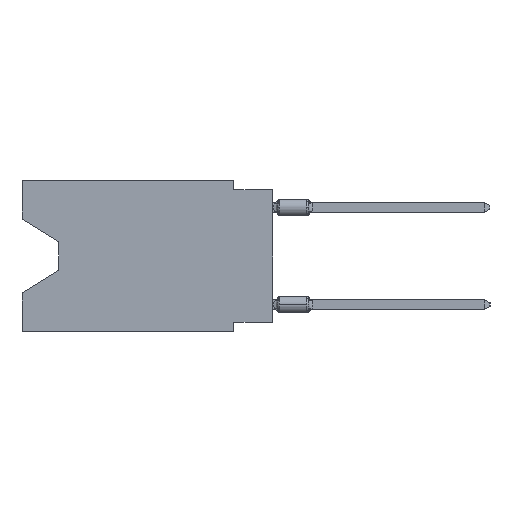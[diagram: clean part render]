
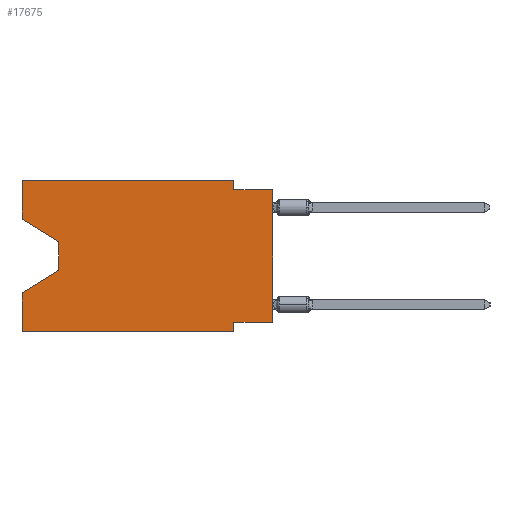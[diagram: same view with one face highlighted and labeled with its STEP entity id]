
A CAD part, left-side view. The second image highlights one B-rep face of the part: STEP entity #17675.
In plain terms, the highlighted planar face has unit normal (-1, 0, 0).
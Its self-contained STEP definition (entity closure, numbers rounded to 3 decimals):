
#400 = CARTESIAN_POINT ( 'NONE',  ( 0., 16.383, -7.36 ) ) ;
#507 = CARTESIAN_POINT ( 'NONE',  ( 0., 16.383, -2.546 ) ) ;
#830 = CARTESIAN_POINT ( 'NONE',  ( 0., 16.383, 0. ) ) ;
#953 = CARTESIAN_POINT ( 'NONE',  ( 0., 0., -0.635 ) ) ;
#1792 = VERTEX_POINT ( 'NONE', #2615 ) ;
#1834 = LINE ( 'NONE', #24312, #50578 ) ;
#1923 = ORIENTED_EDGE ( 'NONE', *, *, #20332, .F. ) ;
#2048 = LINE ( 'NONE', #46701, #47165 ) ;
#2173 = CARTESIAN_POINT ( 'NONE',  ( 0., 13.97, -5.893 ) ) ;
#2421 = VERTEX_POINT ( 'NONE', #4328 ) ;
#2615 = CARTESIAN_POINT ( 'NONE',  ( 0., 16.383, 0. ) ) ;
#3046 = LINE ( 'NONE', #54274, #6098 ) ;
#3304 = VERTEX_POINT ( 'NONE', #55934 ) ;
#4238 = DIRECTION ( 'NONE',  ( 0., 0., -1. ) ) ;
#4328 = CARTESIAN_POINT ( 'NONE',  ( 0., 2.54, -9.271 ) ) ;
#4760 = DIRECTION ( 'NONE',  ( 0., 0., 1. ) ) ;
#5270 = EDGE_CURVE ( 'NONE', #3304, #9733, #3046, .T. ) ;
#6098 = VECTOR ( 'NONE', #26111, 1000. ) ;
#6349 = EDGE_CURVE ( 'NONE', #2421, #26144, #16828, .T. ) ;
#6357 = CARTESIAN_POINT ( 'NONE',  ( 0., 2.54, -9.906 ) ) ;
#8248 = CARTESIAN_POINT ( 'NONE',  ( 0., 16.383, -9.906 ) ) ;
#8907 = EDGE_CURVE ( 'NONE', #13783, #26144, #40299, .T. ) ;
#9733 = VERTEX_POINT ( 'NONE', #2173 ) ;
#11800 = EDGE_CURVE ( 'NONE', #40457, #2421, #2048, .T. ) ;
#12446 = DIRECTION ( 'NONE',  ( 0., -1., 0. ) ) ;
#13056 = CARTESIAN_POINT ( 'NONE',  ( 0., 0., -9.271 ) ) ;
#13783 = VERTEX_POINT ( 'NONE', #56507 ) ;
#14037 = CARTESIAN_POINT ( 'NONE',  ( 0., 16.383, 0. ) ) ;
#14613 = PLANE ( 'NONE',  #41885 ) ;
#14623 = LINE ( 'NONE', #14037, #58030 ) ;
#14653 = DIRECTION ( 'NONE',  ( 0., 1., 0. ) ) ;
#14740 = VERTEX_POINT ( 'NONE', #26604 ) ;
#14767 = VECTOR ( 'NONE', #42408, 1000. ) ;
#15304 = DIRECTION ( 'NONE',  ( 0., 0., 1. ) ) ;
#15509 = EDGE_CURVE ( 'NONE', #1792, #32049, #58820, .T. ) ;
#15875 = CARTESIAN_POINT ( 'NONE',  ( 0., 16.383, 0. ) ) ;
#16316 = VERTEX_POINT ( 'NONE', #26539 ) ;
#16598 = LINE ( 'NONE', #26487, #50656 ) ;
#16828 = LINE ( 'NONE', #25527, #14767 ) ;
#17108 = CARTESIAN_POINT ( 'NONE',  ( 0., 2.54, 0. ) ) ;
#17675 = ADVANCED_FACE ( 'NONE', ( #46363 ), #14613, .F. ) ;
#18218 = DIRECTION ( 'NONE',  ( 0., 0., -1. ) ) ;
#19135 = VECTOR ( 'NONE', #34436, 1000. ) ;
#19222 = DIRECTION ( 'NONE',  ( 0., -1., 0. ) ) ;
#19463 = EDGE_CURVE ( 'NONE', #9733, #44950, #16598, .T. ) ;
#20332 = EDGE_CURVE ( 'NONE', #26983, #1792, #43433, .T. ) ;
#21745 = ORIENTED_EDGE ( 'NONE', *, *, #48545, .F. ) ;
#23669 = EDGE_CURVE ( 'NONE', #40457, #14740, #1834, .T. ) ;
#24005 = EDGE_LOOP ( 'NONE', ( #36872, #46896, #35415, #21745, #49447, #27276, #43816, #47415, #53205, #27104, #34881, #1923 ) ) ;
#24312 = CARTESIAN_POINT ( 'NONE',  ( 0., 0., 0. ) ) ;
#25527 = CARTESIAN_POINT ( 'NONE',  ( 0., 2.54, -9.906 ) ) ;
#25591 = DIRECTION ( 'NONE',  ( 0., 0.855, -0.519 ) ) ;
#26111 = DIRECTION ( 'NONE',  ( 0., 0., -1. ) ) ;
#26144 = VERTEX_POINT ( 'NONE', #6357 ) ;
#26487 = CARTESIAN_POINT ( 'NONE',  ( 0., 13.97, -5.893 ) ) ;
#26539 = CARTESIAN_POINT ( 'NONE',  ( 0., 2.54, -0.635 ) ) ;
#26604 = CARTESIAN_POINT ( 'NONE',  ( 0., 0., -0.635 ) ) ;
#26983 = VERTEX_POINT ( 'NONE', #42974 ) ;
#27002 = LINE ( 'NONE', #17108, #46323 ) ;
#27104 = ORIENTED_EDGE ( 'NONE', *, *, #31969, .F. ) ;
#27276 = ORIENTED_EDGE ( 'NONE', *, *, #6349, .F. ) ;
#27596 = CARTESIAN_POINT ( 'NONE',  ( 0., 2.54, 0. ) ) ;
#31969 = EDGE_CURVE ( 'NONE', #32049, #16316, #27002, .T. ) ;
#32049 = VERTEX_POINT ( 'NONE', #27596 ) ;
#32718 = VECTOR ( 'NONE', #12446, 1000. ) ;
#34436 = DIRECTION ( 'NONE',  ( 0., 0., 1. ) ) ;
#34837 = CARTESIAN_POINT ( 'NONE',  ( 0., 16.383, 0. ) ) ;
#34881 = ORIENTED_EDGE ( 'NONE', *, *, #15509, .F. ) ;
#35113 = VECTOR ( 'NONE', #58217, 1000. ) ;
#35415 = ORIENTED_EDGE ( 'NONE', *, *, #19463, .T. ) ;
#36872 = ORIENTED_EDGE ( 'NONE', *, *, #42463, .T. ) ;
#40299 = LINE ( 'NONE', #8248, #32718 ) ;
#40457 = VERTEX_POINT ( 'NONE', #13056 ) ;
#41560 = LINE ( 'NONE', #507, #48141 ) ;
#41885 = AXIS2_PLACEMENT_3D ( 'NONE', #830, #54481, #18218 ) ;
#42408 = DIRECTION ( 'NONE',  ( 0., 0., -1. ) ) ;
#42463 = EDGE_CURVE ( 'NONE', #26983, #3304, #41560, .T. ) ;
#42974 = CARTESIAN_POINT ( 'NONE',  ( 0., 16.383, -2.546 ) ) ;
#43433 = LINE ( 'NONE', #15875, #19135 ) ;
#43816 = ORIENTED_EDGE ( 'NONE', *, *, #11800, .F. ) ;
#44950 = VERTEX_POINT ( 'NONE', #400 ) ;
#46323 = VECTOR ( 'NONE', #4238, 1000. ) ;
#46363 = FACE_OUTER_BOUND ( 'NONE', #24005, .T. ) ;
#46701 = CARTESIAN_POINT ( 'NONE',  ( 0., 0., -9.271 ) ) ;
#46770 = LINE ( 'NONE', #953, #49103 ) ;
#46896 = ORIENTED_EDGE ( 'NONE', *, *, #5270, .T. ) ;
#47165 = VECTOR ( 'NONE', #14653, 1000. ) ;
#47415 = ORIENTED_EDGE ( 'NONE', *, *, #23669, .T. ) ;
#48141 = VECTOR ( 'NONE', #51423, 1000. ) ;
#48545 = EDGE_CURVE ( 'NONE', #13783, #44950, #14623, .T. ) ;
#49103 = VECTOR ( 'NONE', #19222, 1000. ) ;
#49447 = ORIENTED_EDGE ( 'NONE', *, *, #8907, .T. ) ;
#50578 = VECTOR ( 'NONE', #15304, 1000. ) ;
#50656 = VECTOR ( 'NONE', #25591, 1000. ) ;
#51423 = DIRECTION ( 'NONE',  ( 0., -0.855, -0.519 ) ) ;
#52848 = EDGE_CURVE ( 'NONE', #16316, #14740, #46770, .T. ) ;
#53205 = ORIENTED_EDGE ( 'NONE', *, *, #52848, .F. ) ;
#54274 = CARTESIAN_POINT ( 'NONE',  ( 0., 13.97, -4.013 ) ) ;
#54481 = DIRECTION ( 'NONE',  ( 1., 0., 0. ) ) ;
#55934 = CARTESIAN_POINT ( 'NONE',  ( 0., 13.97, -4.013 ) ) ;
#56507 = CARTESIAN_POINT ( 'NONE',  ( 0., 16.383, -9.906 ) ) ;
#58030 = VECTOR ( 'NONE', #4760, 1000. ) ;
#58217 = DIRECTION ( 'NONE',  ( 0., -1., 0. ) ) ;
#58820 = LINE ( 'NONE', #34837, #35113 ) ;
